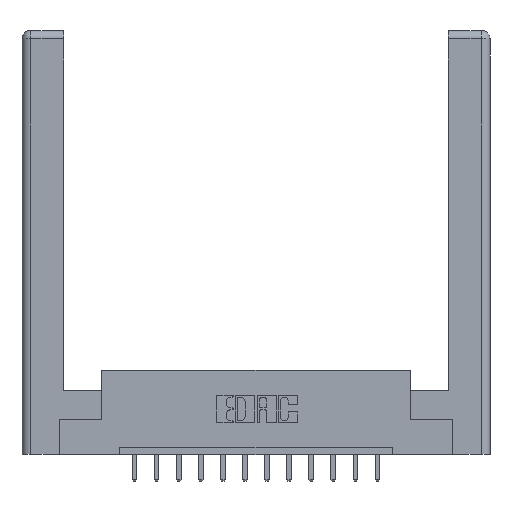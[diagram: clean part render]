
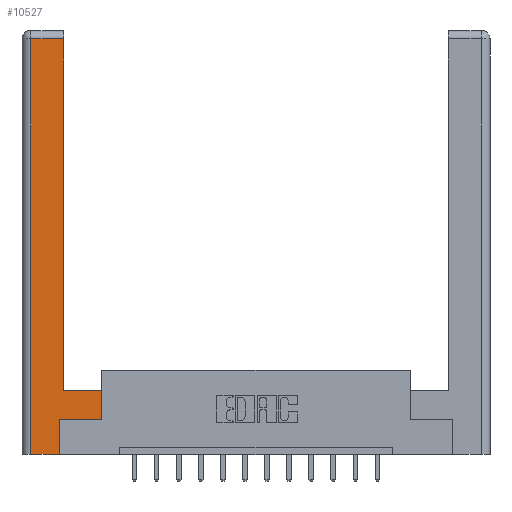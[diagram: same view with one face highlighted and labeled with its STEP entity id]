
A CAD part, top view. The second image highlights one B-rep face of the part: STEP entity #10527.
In plain terms, the highlighted planar face has unit normal (0, 0, 1).
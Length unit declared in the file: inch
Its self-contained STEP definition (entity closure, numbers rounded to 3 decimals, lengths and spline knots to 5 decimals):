
#5 = LINE ( 'NONE', #1917, #6016 ) ;
#154 = EDGE_CURVE ( 'NONE', #13450, #14327, #4498, .T. ) ;
#185 = VERTEX_POINT ( 'NONE', #11311 ) ;
#191 = VECTOR ( 'NONE', #8454, 39.37008 ) ;
#321 = EDGE_CURVE ( 'NONE', #185, #6897, #5, .T. ) ;
#773 = ORIENTED_EDGE ( 'NONE', *, *, #3338, .T. ) ;
#1253 = DIRECTION ( 'NONE',  ( 0., 0., -1. ) ) ;
#1258 = ORIENTED_EDGE ( 'NONE', *, *, #321, .T. ) ;
#1386 = CARTESIAN_POINT ( 'NONE',  ( 0.295, 2.94, 0. ) ) ;
#1461 = CARTESIAN_POINT ( 'NONE',  ( 0.565, 0.45, 0. ) ) ;
#1917 = CARTESIAN_POINT ( 'NONE',  ( 0.265, 0., 0. ) ) ;
#1940 = EDGE_CURVE ( 'NONE', #8487, #7743, #15544, .T. ) ;
#2191 = EDGE_CURVE ( 'NONE', #11860, #13450, #5215, .T. ) ;
#3027 = VECTOR ( 'NONE', #5753, 39.37008 ) ;
#3228 = FACE_OUTER_BOUND ( 'NONE', #14937, .T. ) ;
#3338 = EDGE_CURVE ( 'NONE', #7743, #8697, #3372, .T. ) ;
#3372 = LINE ( 'NONE', #7241, #191 ) ;
#3632 = ORIENTED_EDGE ( 'NONE', *, *, #1940, .T. ) ;
#3659 = CARTESIAN_POINT ( 'NONE',  ( 0.265, 0., 0. ) ) ;
#3703 = DIRECTION ( 'NONE',  ( -1., 0., 0. ) ) ;
#4175 = EDGE_CURVE ( 'NONE', #6897, #11860, #10701, .T. ) ;
#4275 = CARTESIAN_POINT ( 'NONE',  ( 0.0615, 2.94, 0. ) ) ;
#4498 = LINE ( 'NONE', #10887, #4671 ) ;
#4671 = VECTOR ( 'NONE', #9743, 39.37008 ) ;
#4817 = CARTESIAN_POINT ( 'NONE',  ( 0.565, 0.245, 0. ) ) ;
#5215 = LINE ( 'NONE', #4817, #6894 ) ;
#5712 = CARTESIAN_POINT ( 'NONE',  ( 0.265, 0.245, 0. ) ) ;
#5753 = DIRECTION ( 'NONE',  ( 0., -1., 0. ) ) ;
#5859 = LINE ( 'NONE', #12944, #3027 ) ;
#6016 = VECTOR ( 'NONE', #6598, 39.37008 ) ;
#6391 = AXIS2_PLACEMENT_3D ( 'NONE', #11095, #1253, #7398 ) ;
#6598 = DIRECTION ( 'NONE',  ( 1., 0., 0. ) ) ;
#6894 = VECTOR ( 'NONE', #8481, 39.37008 ) ;
#6897 = VERTEX_POINT ( 'NONE', #3659 ) ;
#7196 = CARTESIAN_POINT ( 'NONE',  ( 0.295, 0.45, 0. ) ) ;
#7241 = CARTESIAN_POINT ( 'NONE',  ( 0.0615, 2.94, 0. ) ) ;
#7299 = VECTOR ( 'NONE', #13128, 39.37008 ) ;
#7398 = DIRECTION ( 'NONE',  ( -1., 0., 0. ) ) ;
#7551 = ORIENTED_EDGE ( 'NONE', *, *, #10585, .T. ) ;
#7743 = VERTEX_POINT ( 'NONE', #1386 ) ;
#8454 = DIRECTION ( 'NONE',  ( -1., 0., 0. ) ) ;
#8468 = CARTESIAN_POINT ( 'NONE',  ( 0.265, 0.245, 0. ) ) ;
#8481 = DIRECTION ( 'NONE',  ( 1., 0., 0. ) ) ;
#8487 = VERTEX_POINT ( 'NONE', #13622 ) ;
#8583 = CARTESIAN_POINT ( 'NONE',  ( 0.295, 3., 0. ) ) ;
#8697 = VERTEX_POINT ( 'NONE', #4275 ) ;
#9743 = DIRECTION ( 'NONE',  ( 0., 1., 0. ) ) ;
#10220 = ORIENTED_EDGE ( 'NONE', *, *, #2191, .T. ) ;
#10512 = VECTOR ( 'NONE', #10751, 39.37008 ) ;
#10527 = ADVANCED_FACE ( 'NONE', ( #3228 ), #13317, .F. ) ;
#10585 = EDGE_CURVE ( 'NONE', #8697, #185, #5859, .T. ) ;
#10701 = LINE ( 'NONE', #8468, #7299 ) ;
#10751 = DIRECTION ( 'NONE',  ( 0., 1., 0. ) ) ;
#10887 = CARTESIAN_POINT ( 'NONE',  ( 0.565, 0.45, 0. ) ) ;
#11095 = CARTESIAN_POINT ( 'NONE',  ( 0., 0., 0. ) ) ;
#11266 = ORIENTED_EDGE ( 'NONE', *, *, #11270, .T. ) ;
#11270 = EDGE_CURVE ( 'NONE', #14327, #8487, #14291, .T. ) ;
#11311 = CARTESIAN_POINT ( 'NONE',  ( 0.0615, 0., 0. ) ) ;
#11561 = ORIENTED_EDGE ( 'NONE', *, *, #154, .T. ) ;
#11860 = VERTEX_POINT ( 'NONE', #5712 ) ;
#12008 = ORIENTED_EDGE ( 'NONE', *, *, #4175, .T. ) ;
#12944 = CARTESIAN_POINT ( 'NONE',  ( 0.0615, 0., 0. ) ) ;
#12959 = CARTESIAN_POINT ( 'NONE',  ( 0.565, 0.245, 0. ) ) ;
#13128 = DIRECTION ( 'NONE',  ( 0., 1., 0. ) ) ;
#13317 = PLANE ( 'NONE',  #6391 ) ;
#13450 = VERTEX_POINT ( 'NONE', #12959 ) ;
#13622 = CARTESIAN_POINT ( 'NONE',  ( 0.295, 0.45, 0. ) ) ;
#14291 = LINE ( 'NONE', #7196, #14865 ) ;
#14327 = VERTEX_POINT ( 'NONE', #1461 ) ;
#14865 = VECTOR ( 'NONE', #3703, 39.37008 ) ;
#14937 = EDGE_LOOP ( 'NONE', ( #3632, #773, #7551, #1258, #12008, #10220, #11561, #11266 ) ) ;
#15544 = LINE ( 'NONE', #8583, #10512 ) ;
